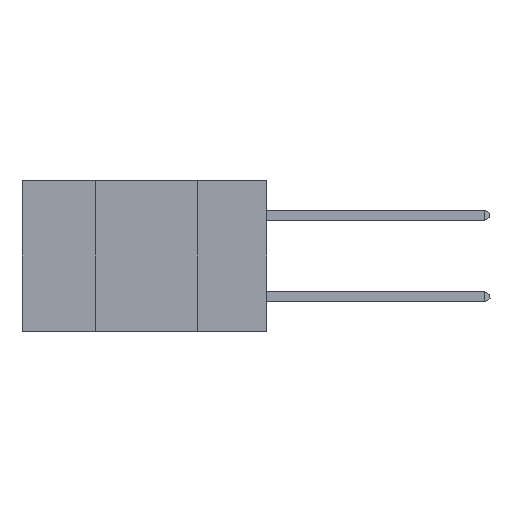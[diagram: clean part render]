
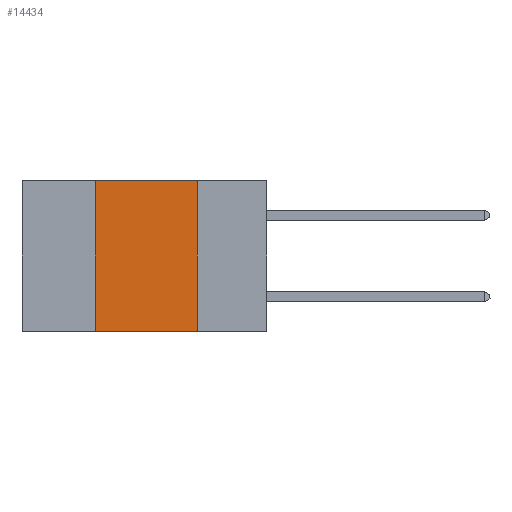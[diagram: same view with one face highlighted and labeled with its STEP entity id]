
A CAD part, left-side view. The second image highlights one B-rep face of the part: STEP entity #14434.
In plain terms, the highlighted planar face has unit normal (-1, 0, 0).
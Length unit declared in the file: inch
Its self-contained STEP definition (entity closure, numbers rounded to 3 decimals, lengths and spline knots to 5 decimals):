
#250 = DIRECTION ( 'NONE',  ( 0., -1., 0. ) ) ;
#514 = DIRECTION ( 'NONE',  ( 1., 0., 0. ) ) ;
#596 = ORIENTED_EDGE ( 'NONE', *, *, #12522, .T. ) ;
#1102 = CARTESIAN_POINT ( 'NONE',  ( 0., 0.6, 0. ) ) ;
#1525 = VERTEX_POINT ( 'NONE', #5777 ) ;
#1902 = VERTEX_POINT ( 'NONE', #19765 ) ;
#2297 = PLANE ( 'NONE',  #15504 ) ;
#4123 = VECTOR ( 'NONE', #21287, 39.37008 ) ;
#4392 = ORIENTED_EDGE ( 'NONE', *, *, #19596, .F. ) ;
#4517 = EDGE_CURVE ( 'NONE', #20666, #1902, #14564, .T. ) ;
#5001 = ORIENTED_EDGE ( 'NONE', *, *, #23051, .F. ) ;
#5099 = CARTESIAN_POINT ( 'NONE',  ( 0., 0.42, -0.37 ) ) ;
#5288 = VECTOR ( 'NONE', #21275, 39.37008 ) ;
#5777 = CARTESIAN_POINT ( 'NONE',  ( 0., 0.17, -0.37 ) ) ;
#7841 = FACE_OUTER_BOUND ( 'NONE', #22734, .T. ) ;
#7980 = CARTESIAN_POINT ( 'NONE',  ( 0., 0.6, 0. ) ) ;
#8738 = CARTESIAN_POINT ( 'NONE',  ( 0., 0.17, 0. ) ) ;
#9234 = VECTOR ( 'NONE', #17837, 39.37008 ) ;
#9802 = LINE ( 'NONE', #8738, #9234 ) ;
#10379 = CARTESIAN_POINT ( 'NONE',  ( 0., 0.42, 0. ) ) ;
#12522 = EDGE_CURVE ( 'NONE', #17865, #1525, #15431, .T. ) ;
#13551 = DIRECTION ( 'NONE',  ( 0., 0., -1. ) ) ;
#14434 = ADVANCED_FACE ( 'NONE', ( #7841 ), #2297, .F. ) ;
#14564 = LINE ( 'NONE', #1102, #5288 ) ;
#15431 = LINE ( 'NONE', #22285, #19668 ) ;
#15504 = AXIS2_PLACEMENT_3D ( 'NONE', #7980, #514, #13551 ) ;
#17837 = DIRECTION ( 'NONE',  ( 0., 0., -1. ) ) ;
#17865 = VERTEX_POINT ( 'NONE', #5099 ) ;
#18838 = LINE ( 'NONE', #19494, #4123 ) ;
#19097 = ORIENTED_EDGE ( 'NONE', *, *, #4517, .F. ) ;
#19494 = CARTESIAN_POINT ( 'NONE',  ( 0., 0.42, 0. ) ) ;
#19596 = EDGE_CURVE ( 'NONE', #1902, #1525, #9802, .T. ) ;
#19668 = VECTOR ( 'NONE', #250, 39.37008 ) ;
#19765 = CARTESIAN_POINT ( 'NONE',  ( 0., 0.17, 0. ) ) ;
#20666 = VERTEX_POINT ( 'NONE', #10379 ) ;
#21275 = DIRECTION ( 'NONE',  ( 0., -1., 0. ) ) ;
#21287 = DIRECTION ( 'NONE',  ( 0., 0., 1. ) ) ;
#22285 = CARTESIAN_POINT ( 'NONE',  ( 0., 0.6, -0.37 ) ) ;
#22734 = EDGE_LOOP ( 'NONE', ( #4392, #19097, #5001, #596 ) ) ;
#23051 = EDGE_CURVE ( 'NONE', #17865, #20666, #18838, .T. ) ;
